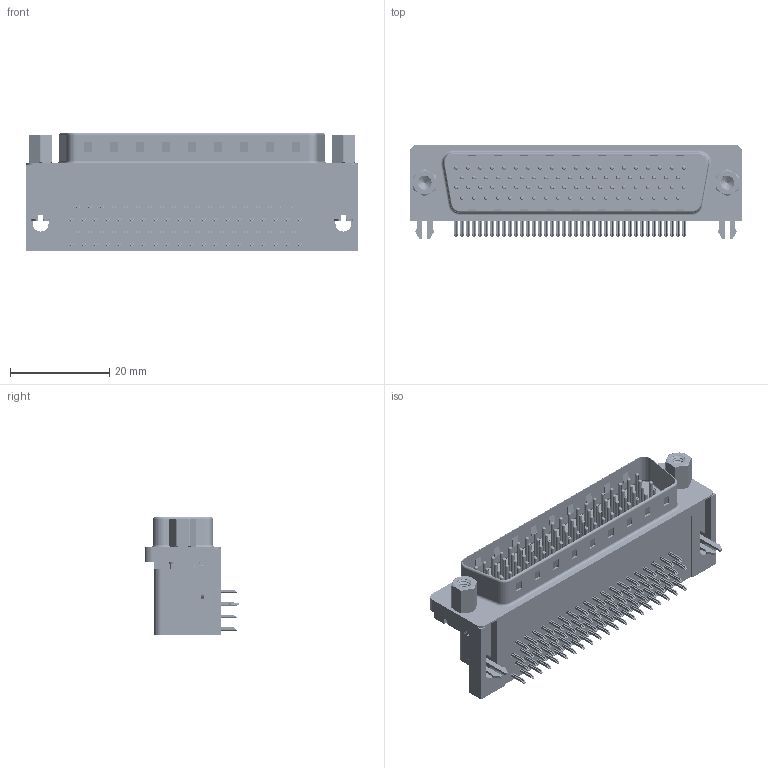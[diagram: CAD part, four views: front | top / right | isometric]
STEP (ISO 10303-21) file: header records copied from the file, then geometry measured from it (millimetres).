
FILE_DESCRIPTION (( 'STEP AP203' ), '1' );
FILE_NAME ('633-078-663-033.STEP', '2018-09-08T15:33:51', ( '' ), ( '' ), 'SwSTEP 2.0', 'SolidWorks 2016', '' );
FILE_SCHEMA (( 'CONFIG_CONTROL_DESIGN' ));
Length unit declared in the file: millimetre
Products named in the file (10): 633 Contact Top 78; 633 2 Prong Board Lock_78 Contact; 633 4-40 Threaded Rivet; 633 4-40 Hex Standoff; 633 Housing_78 Contact; 633-078-663-033; 633 Shell_78 Contact; 633 Contact Bottom_78 Contact; 633 Contact Middle_78 Contact; 633 Contact Top_78 Contact
Assembly tree (86 placements, depth 2):
  633-078-663-033
    633 Housing_78 Contact
    633 Shell_78 Contact
    633 Contact Bottom_78 Contact  x19
    633 Contact Middle_78 Contact  x20
    633 Contact Top_78 Contact  x19
    633 Contact Top 78  x20
    633 2 Prong Board Lock_78 Contact  x2
    633 4-40 Threaded Rivet  x2
    633 4-40 Hex Standoff  x2
Bounding box: 67 x 19.1 x 23.8 mm (x, y, z)
Volume: 14814.7 mm3; surface area: 16811 mm2
Topology: 86 solids, 86 shells, 6436 faces, 15862 edges, 9761 vertices
Faces by surface type: plane 4035, cylinder 1850, torus 499, cone 34, bspline 18
Entity records: 46245 total; most frequent: CARTESIAN_POINT 11045, DIRECTION 6736, ORIENTED_EDGE 6488, EDGE_CURVE 3244, VECTOR 2298, LINE 2298, AXIS2_PLACEMENT_3D 2219, VERTEX_POINT 2097
